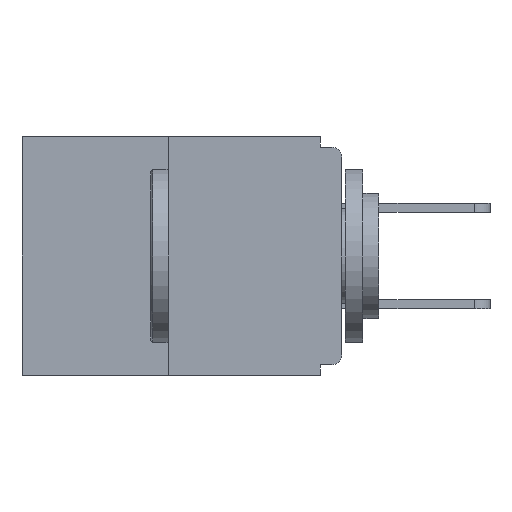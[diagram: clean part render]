
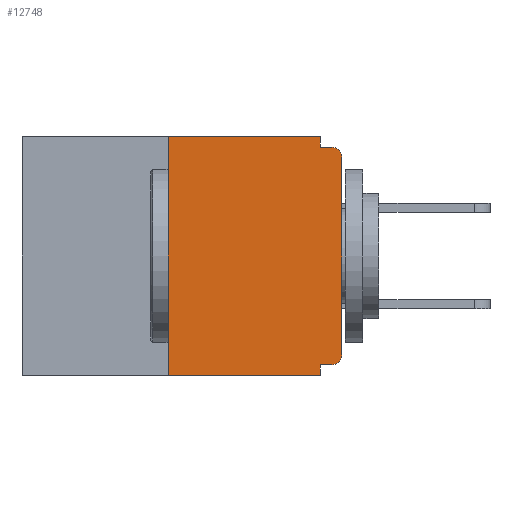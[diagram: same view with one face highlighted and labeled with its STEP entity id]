
A CAD part, left-side view. The second image highlights one B-rep face of the part: STEP entity #12748.
In plain terms, the highlighted planar face has unit normal (-1, 0, 0).
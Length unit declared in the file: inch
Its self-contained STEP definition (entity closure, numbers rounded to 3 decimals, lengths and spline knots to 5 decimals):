
#62 = EDGE_CURVE ( 'NONE', #6152, #12022, #15247, .T. ) ;
#167 = DIRECTION ( 'NONE',  ( 1., 0., 0. ) ) ;
#545 = CARTESIAN_POINT ( 'NONE',  ( 0., 0.031, -0.328 ) ) ;
#672 = DIRECTION ( 'NONE',  ( -1., 0., 0. ) ) ;
#843 = VERTEX_POINT ( 'NONE', #7295 ) ;
#940 = CARTESIAN_POINT ( 'NONE',  ( 0., 0.46, -0.343 ) ) ;
#1123 = CARTESIAN_POINT ( 'NONE',  ( 0., 0.015, -0.328 ) ) ;
#1277 = DIRECTION ( 'NONE',  ( 0., 0., -1. ) ) ;
#1443 = DIRECTION ( 'NONE',  ( -1., 0., 0. ) ) ;
#1703 = VECTOR ( 'NONE', #9972, 39.37008 ) ;
#1924 = LINE ( 'NONE', #6907, #13867 ) ;
#1973 = EDGE_CURVE ( 'NONE', #5705, #6079, #8065, .T. ) ;
#2233 = VECTOR ( 'NONE', #1277, 39.37008 ) ;
#2380 = FACE_OUTER_BOUND ( 'NONE', #15863, .T. ) ;
#2465 = ORIENTED_EDGE ( 'NONE', *, *, #9421, .F. ) ;
#2474 = ORIENTED_EDGE ( 'NONE', *, *, #62, .F. ) ;
#3294 = CARTESIAN_POINT ( 'NONE',  ( 0., 0.25, 0. ) ) ;
#3490 = LINE ( 'NONE', #940, #14591 ) ;
#3560 = DIRECTION ( 'NONE',  ( 0., -1., 0. ) ) ;
#3712 = CARTESIAN_POINT ( 'NONE',  ( 0., 0.46, 0. ) ) ;
#4114 = LINE ( 'NONE', #14980, #2233 ) ;
#4154 = AXIS2_PLACEMENT_3D ( 'NONE', #9748, #167, #4315 ) ;
#4225 = CARTESIAN_POINT ( 'NONE',  ( 0., 0.015, -0.03 ) ) ;
#4266 = LINE ( 'NONE', #4613, #1703 ) ;
#4283 = ORIENTED_EDGE ( 'NONE', *, *, #10088, .T. ) ;
#4315 = DIRECTION ( 'NONE',  ( 0., 0., -1. ) ) ;
#4387 = VERTEX_POINT ( 'NONE', #5710 ) ;
#4562 = AXIS2_PLACEMENT_3D ( 'NONE', #15304, #1443, #5954 ) ;
#4613 = CARTESIAN_POINT ( 'NONE',  ( 0., 0., -0.328 ) ) ;
#4698 = EDGE_CURVE ( 'NONE', #843, #16589, #3490, .T. ) ;
#5152 = ORIENTED_EDGE ( 'NONE', *, *, #4698, .T. ) ;
#5473 = CIRCLE ( 'NONE', #13883, 0.015 ) ;
#5705 = VERTEX_POINT ( 'NONE', #1123 ) ;
#5710 = CARTESIAN_POINT ( 'NONE',  ( 0., 0.25, 0. ) ) ;
#5954 = DIRECTION ( 'NONE',  ( 0., 0., -1. ) ) ;
#6079 = VERTEX_POINT ( 'NONE', #15961 ) ;
#6136 = EDGE_CURVE ( 'NONE', #4387, #11180, #16202, .T. ) ;
#6152 = VERTEX_POINT ( 'NONE', #15796 ) ;
#6179 = ORIENTED_EDGE ( 'NONE', *, *, #6136, .F. ) ;
#6336 = VERTEX_POINT ( 'NONE', #545 ) ;
#6907 = CARTESIAN_POINT ( 'NONE',  ( 0., 0., 0. ) ) ;
#7295 = CARTESIAN_POINT ( 'NONE',  ( 0., 0.25, -0.343 ) ) ;
#7593 = ORIENTED_EDGE ( 'NONE', *, *, #1973, .T. ) ;
#8065 = CIRCLE ( 'NONE', #4562, 0.015 ) ;
#8513 = CARTESIAN_POINT ( 'NONE',  ( 0., 0., -0.015 ) ) ;
#8545 = VECTOR ( 'NONE', #12891, 39.37008 ) ;
#9052 = CARTESIAN_POINT ( 'NONE',  ( 0., 0.031, -0.343 ) ) ;
#9303 = VECTOR ( 'NONE', #11067, 39.37008 ) ;
#9421 = EDGE_CURVE ( 'NONE', #11180, #6152, #12297, .T. ) ;
#9748 = CARTESIAN_POINT ( 'NONE',  ( 0., 0.46, 0. ) ) ;
#9972 = DIRECTION ( 'NONE',  ( 0., 1., 0. ) ) ;
#10088 = EDGE_CURVE ( 'NONE', #15277, #12022, #5473, .T. ) ;
#10114 = CARTESIAN_POINT ( 'NONE',  ( 0., 0.031, 0. ) ) ;
#10238 = ORIENTED_EDGE ( 'NONE', *, *, #13350, .F. ) ;
#10954 = DIRECTION ( 'NONE',  ( 0., 0., 1. ) ) ;
#11067 = DIRECTION ( 'NONE',  ( 0., -1., 0. ) ) ;
#11180 = VERTEX_POINT ( 'NONE', #10114 ) ;
#11718 = DIRECTION ( 'NONE',  ( 0., -1., 0. ) ) ;
#12022 = VERTEX_POINT ( 'NONE', #13786 ) ;
#12297 = LINE ( 'NONE', #17223, #14011 ) ;
#12421 = ORIENTED_EDGE ( 'NONE', *, *, #17438, .F. ) ;
#12748 = ADVANCED_FACE ( 'NONE', ( #2380 ), #13706, .F. ) ;
#12891 = DIRECTION ( 'NONE',  ( 0., 0., 1. ) ) ;
#13043 = VECTOR ( 'NONE', #11718, 39.37008 ) ;
#13324 = DIRECTION ( 'NONE',  ( 0., 0., -1. ) ) ;
#13349 = EDGE_CURVE ( 'NONE', #843, #4387, #15154, .T. ) ;
#13350 = EDGE_CURVE ( 'NONE', #5705, #6336, #4266, .T. ) ;
#13700 = ORIENTED_EDGE ( 'NONE', *, *, #13349, .F. ) ;
#13706 = PLANE ( 'NONE',  #4154 ) ;
#13786 = CARTESIAN_POINT ( 'NONE',  ( 0., 0.015, -0.015 ) ) ;
#13847 = DIRECTION ( 'NONE',  ( 0., 0., -1. ) ) ;
#13867 = VECTOR ( 'NONE', #10954, 39.37008 ) ;
#13883 = AXIS2_PLACEMENT_3D ( 'NONE', #4225, #672, #13847 ) ;
#13967 = EDGE_CURVE ( 'NONE', #6079, #15277, #1924, .T. ) ;
#14011 = VECTOR ( 'NONE', #13324, 39.37008 ) ;
#14591 = VECTOR ( 'NONE', #3560, 39.37008 ) ;
#14980 = CARTESIAN_POINT ( 'NONE',  ( 0., 0.031, -0.343 ) ) ;
#15154 = LINE ( 'NONE', #3294, #8545 ) ;
#15247 = LINE ( 'NONE', #8513, #9303 ) ;
#15277 = VERTEX_POINT ( 'NONE', #15993 ) ;
#15304 = CARTESIAN_POINT ( 'NONE',  ( 0., 0.015, -0.313 ) ) ;
#15796 = CARTESIAN_POINT ( 'NONE',  ( 0., 0.031, -0.015 ) ) ;
#15863 = EDGE_LOOP ( 'NONE', ( #6179, #13700, #5152, #12421, #10238, #7593, #15967, #4283, #2474, #2465 ) ) ;
#15961 = CARTESIAN_POINT ( 'NONE',  ( 0., 0., -0.313 ) ) ;
#15967 = ORIENTED_EDGE ( 'NONE', *, *, #13967, .T. ) ;
#15993 = CARTESIAN_POINT ( 'NONE',  ( 0., 0., -0.03 ) ) ;
#16202 = LINE ( 'NONE', #3712, #13043 ) ;
#16589 = VERTEX_POINT ( 'NONE', #9052 ) ;
#17223 = CARTESIAN_POINT ( 'NONE',  ( 0., 0.031, 0. ) ) ;
#17438 = EDGE_CURVE ( 'NONE', #6336, #16589, #4114, .T. ) ;
